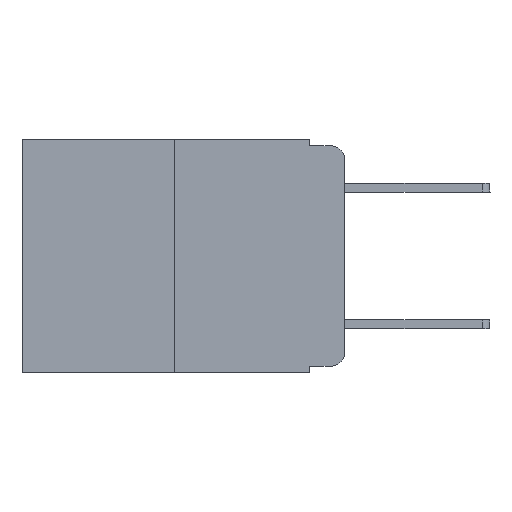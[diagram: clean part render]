
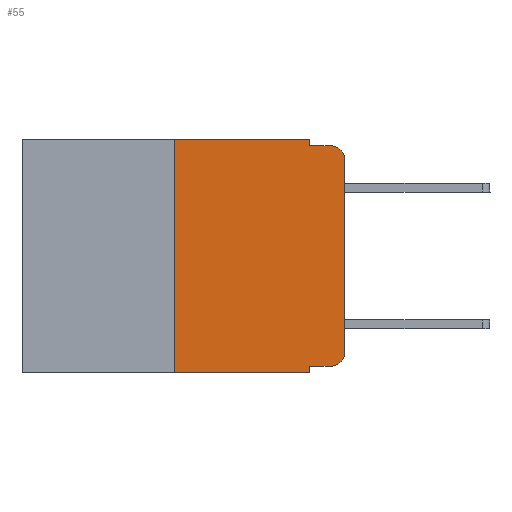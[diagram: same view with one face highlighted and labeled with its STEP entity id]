
A CAD part, left-side view. The second image highlights one B-rep face of the part: STEP entity #55.
In plain terms, the highlighted planar face has unit normal (-1, 0, 0).
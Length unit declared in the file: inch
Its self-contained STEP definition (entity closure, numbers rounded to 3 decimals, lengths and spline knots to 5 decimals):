
#55 = ADVANCED_FACE ( 'NONE', ( #8828 ), #3147, .F. ) ;
#513 = ORIENTED_EDGE ( 'NONE', *, *, #9046, .T. ) ;
#754 = EDGE_CURVE ( 'NONE', #4234, #3669, #5045, .T. ) ;
#1007 = ORIENTED_EDGE ( 'NONE', *, *, #8216, .T. ) ;
#1023 = ORIENTED_EDGE ( 'NONE', *, *, #1926, .F. ) ;
#1025 = DIRECTION ( 'NONE',  ( 0., 0., 1. ) ) ;
#1075 = CARTESIAN_POINT ( 'NONE',  ( 0., 0.051, 0. ) ) ;
#1666 = CARTESIAN_POINT ( 'NONE',  ( 0., 0.051, -0.333 ) ) ;
#1711 = CARTESIAN_POINT ( 'NONE',  ( 0., 0.02, -0.313 ) ) ;
#1750 = ORIENTED_EDGE ( 'NONE', *, *, #7103, .F. ) ;
#1782 = ORIENTED_EDGE ( 'NONE', *, *, #10590, .F. ) ;
#1926 = EDGE_CURVE ( 'NONE', #12898, #6146, #2293, .T. ) ;
#2291 = CIRCLE ( 'NONE', #10901, 0.02 ) ;
#2293 = LINE ( 'NONE', #4532, #11231 ) ;
#2934 = EDGE_CURVE ( 'NONE', #12848, #4234, #2291, .T. ) ;
#3026 = CARTESIAN_POINT ( 'NONE',  ( 0., 0.473, -0.343 ) ) ;
#3147 = PLANE ( 'NONE',  #9310 ) ;
#3210 = CARTESIAN_POINT ( 'NONE',  ( 0., 0.051, -0.333 ) ) ;
#3300 = DIRECTION ( 'NONE',  ( 0., -1., 0. ) ) ;
#3318 = DIRECTION ( 'NONE',  ( 0., 0., -1. ) ) ;
#3365 = LINE ( 'NONE', #5692, #4386 ) ;
#3471 = CARTESIAN_POINT ( 'NONE',  ( 0., 0.02, -0.333 ) ) ;
#3669 = VERTEX_POINT ( 'NONE', #7366 ) ;
#3767 = CARTESIAN_POINT ( 'NONE',  ( 0., 0.051, -0.343 ) ) ;
#3933 = DIRECTION ( 'NONE',  ( 0., 0., -1. ) ) ;
#3948 = CARTESIAN_POINT ( 'NONE',  ( 0., 0.051, 0. ) ) ;
#4234 = VERTEX_POINT ( 'NONE', #11653 ) ;
#4295 = ORIENTED_EDGE ( 'NONE', *, *, #754, .T. ) ;
#4386 = VECTOR ( 'NONE', #3300, 39.37008 ) ;
#4415 = VECTOR ( 'NONE', #8408, 39.37008 ) ;
#4532 = CARTESIAN_POINT ( 'NONE',  ( 0., 0.25, 0. ) ) ;
#4758 = VERTEX_POINT ( 'NONE', #14468 ) ;
#4931 = VERTEX_POINT ( 'NONE', #1075 ) ;
#5012 = DIRECTION ( 'NONE',  ( -1., 0., 0. ) ) ;
#5045 = LINE ( 'NONE', #13036, #4415 ) ;
#5057 = CARTESIAN_POINT ( 'NONE',  ( 0., 0.02, -0.03 ) ) ;
#5139 = VERTEX_POINT ( 'NONE', #3767 ) ;
#5223 = VERTEX_POINT ( 'NONE', #1666 ) ;
#5309 = LINE ( 'NONE', #3210, #12991 ) ;
#5346 = DIRECTION ( 'NONE',  ( 0., -1., 0. ) ) ;
#5516 = ORIENTED_EDGE ( 'NONE', *, *, #14333, .F. ) ;
#5561 = LINE ( 'NONE', #3026, #13703 ) ;
#5692 = CARTESIAN_POINT ( 'NONE',  ( 0., 0.473, 0. ) ) ;
#6146 = VERTEX_POINT ( 'NONE', #13047 ) ;
#6165 = ORIENTED_EDGE ( 'NONE', *, *, #11506, .F. ) ;
#6209 = LINE ( 'NONE', #7173, #6803 ) ;
#6277 = DIRECTION ( 'NONE',  ( 0., -1., 0. ) ) ;
#6662 = DIRECTION ( 'NONE',  ( 1., 0., 0. ) ) ;
#6717 = VECTOR ( 'NONE', #8517, 39.37008 ) ;
#6803 = VECTOR ( 'NONE', #6277, 39.37008 ) ;
#6913 = ORIENTED_EDGE ( 'NONE', *, *, #7927, .T. ) ;
#7103 = EDGE_CURVE ( 'NONE', #6146, #4931, #3365, .T. ) ;
#7173 = CARTESIAN_POINT ( 'NONE',  ( 0., 0.051, -0.01 ) ) ;
#7232 = LINE ( 'NONE', #3948, #6717 ) ;
#7366 = CARTESIAN_POINT ( 'NONE',  ( 0., 0., -0.03 ) ) ;
#7866 = CARTESIAN_POINT ( 'NONE',  ( 0., 0.051, 0. ) ) ;
#7927 = EDGE_CURVE ( 'NONE', #3669, #10967, #8236, .T. ) ;
#8216 = EDGE_CURVE ( 'NONE', #12898, #5139, #5561, .T. ) ;
#8236 = CIRCLE ( 'NONE', #8481, 0.02 ) ;
#8408 = DIRECTION ( 'NONE',  ( 0., 0., 1. ) ) ;
#8481 = AXIS2_PLACEMENT_3D ( 'NONE', #5057, #10818, #3933 ) ;
#8517 = DIRECTION ( 'NONE',  ( 0., 0., -1. ) ) ;
#8828 = FACE_OUTER_BOUND ( 'NONE', #14526, .T. ) ;
#9046 = EDGE_CURVE ( 'NONE', #5223, #12848, #5309, .T. ) ;
#9310 = AXIS2_PLACEMENT_3D ( 'NONE', #12342, #6662, #14653 ) ;
#9863 = DIRECTION ( 'NONE',  ( 0., -1., 0. ) ) ;
#10187 = LINE ( 'NONE', #7866, #12792 ) ;
#10419 = CARTESIAN_POINT ( 'NONE',  ( 0., 0.25, -0.343 ) ) ;
#10590 = EDGE_CURVE ( 'NONE', #4931, #4758, #7232, .T. ) ;
#10818 = DIRECTION ( 'NONE',  ( -1., 0., 0. ) ) ;
#10901 = AXIS2_PLACEMENT_3D ( 'NONE', #1711, #5012, #12029 ) ;
#10967 = VERTEX_POINT ( 'NONE', #12826 ) ;
#11231 = VECTOR ( 'NONE', #1025, 39.37008 ) ;
#11506 = EDGE_CURVE ( 'NONE', #4758, #10967, #6209, .T. ) ;
#11653 = CARTESIAN_POINT ( 'NONE',  ( 0., 0., -0.313 ) ) ;
#11902 = ORIENTED_EDGE ( 'NONE', *, *, #2934, .T. ) ;
#12029 = DIRECTION ( 'NONE',  ( 0., 0., -1. ) ) ;
#12342 = CARTESIAN_POINT ( 'NONE',  ( 0., 0.473, 0. ) ) ;
#12792 = VECTOR ( 'NONE', #3318, 39.37008 ) ;
#12826 = CARTESIAN_POINT ( 'NONE',  ( 0., 0.02, -0.01 ) ) ;
#12848 = VERTEX_POINT ( 'NONE', #3471 ) ;
#12898 = VERTEX_POINT ( 'NONE', #10419 ) ;
#12991 = VECTOR ( 'NONE', #9863, 39.37008 ) ;
#13036 = CARTESIAN_POINT ( 'NONE',  ( 0., 0., 0. ) ) ;
#13047 = CARTESIAN_POINT ( 'NONE',  ( 0., 0.25, 0. ) ) ;
#13703 = VECTOR ( 'NONE', #5346, 39.37008 ) ;
#14333 = EDGE_CURVE ( 'NONE', #5223, #5139, #10187, .T. ) ;
#14468 = CARTESIAN_POINT ( 'NONE',  ( 0., 0.051, -0.01 ) ) ;
#14526 = EDGE_LOOP ( 'NONE', ( #4295, #6913, #6165, #1782, #1750, #1023, #1007, #5516, #513, #11902 ) ) ;
#14653 = DIRECTION ( 'NONE',  ( 0., 0., -1. ) ) ;
